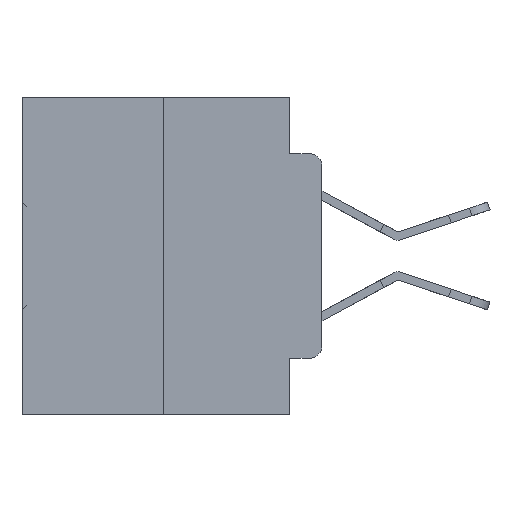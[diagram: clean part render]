
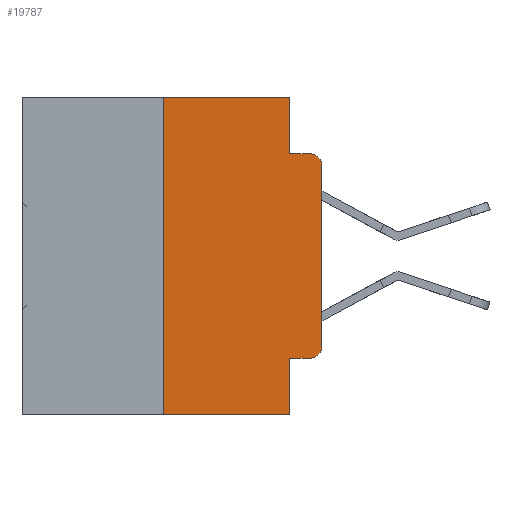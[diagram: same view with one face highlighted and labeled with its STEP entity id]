
A CAD part, left-side view. The second image highlights one B-rep face of the part: STEP entity #19787.
In plain terms, the highlighted planar face has unit normal (-1, 0, 0).
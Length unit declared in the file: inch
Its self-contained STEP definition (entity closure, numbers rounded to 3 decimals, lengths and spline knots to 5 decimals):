
#76 = ORIENTED_EDGE ( 'NONE', *, *, #14428, .T. ) ;
#88 = CARTESIAN_POINT ( 'NONE',  ( 0., 0.051, -0.0885 ) ) ;
#869 = LINE ( 'NONE', #19992, #21057 ) ;
#958 = EDGE_LOOP ( 'NONE', ( #20380, #28626, #30438, #4916, #33759, #33147, #13975, #3211, #12339, #76 ) ) ;
#1133 = VECTOR ( 'NONE', #30900, 39.37008 ) ;
#1187 = CARTESIAN_POINT ( 'NONE',  ( 0., 0.051, 0. ) ) ;
#1416 = DIRECTION ( 'NONE',  ( 0., 0., -1. ) ) ;
#1896 = CARTESIAN_POINT ( 'NONE',  ( 0., 0.02, -0.4115 ) ) ;
#2164 = CARTESIAN_POINT ( 'NONE',  ( 0., 0., -0.3915 ) ) ;
#2449 = CARTESIAN_POINT ( 'NONE',  ( 0., 0.051, 0. ) ) ;
#2727 = DIRECTION ( 'NONE',  ( 0., -1., 0. ) ) ;
#3211 = ORIENTED_EDGE ( 'NONE', *, *, #10693, .F. ) ;
#3385 = CARTESIAN_POINT ( 'NONE',  ( 0., 0.051, -0.4115 ) ) ;
#3514 = VECTOR ( 'NONE', #34036, 39.37008 ) ;
#4916 = ORIENTED_EDGE ( 'NONE', *, *, #24841, .F. ) ;
#5304 = LINE ( 'NONE', #15286, #1133 ) ;
#5607 = CARTESIAN_POINT ( 'NONE',  ( 0., 0.473, -0.5 ) ) ;
#5660 = VERTEX_POINT ( 'NONE', #22393 ) ;
#5994 = AXIS2_PLACEMENT_3D ( 'NONE', #28397, #18089, #31273 ) ;
#7220 = CARTESIAN_POINT ( 'NONE',  ( 0., 0.02, -0.3915 ) ) ;
#7472 = LINE ( 'NONE', #33695, #13221 ) ;
#7655 = DIRECTION ( 'NONE',  ( 0., -1., 0. ) ) ;
#7830 = VERTEX_POINT ( 'NONE', #17586 ) ;
#8299 = EDGE_CURVE ( 'NONE', #16056, #25150, #869, .T. ) ;
#10693 = EDGE_CURVE ( 'NONE', #19736, #5660, #5304, .T. ) ;
#10862 = DIRECTION ( 'NONE',  ( 0., -1., 0. ) ) ;
#11184 = VECTOR ( 'NONE', #10862, 39.37008 ) ;
#11943 = VERTEX_POINT ( 'NONE', #29329 ) ;
#12188 = VERTEX_POINT ( 'NONE', #1896 ) ;
#12197 = EDGE_CURVE ( 'NONE', #22142, #16056, #12635, .T. ) ;
#12215 = EDGE_CURVE ( 'NONE', #23981, #11943, #31503, .T. ) ;
#12339 = ORIENTED_EDGE ( 'NONE', *, *, #21670, .T. ) ;
#12635 = LINE ( 'NONE', #22845, #28660 ) ;
#13221 = VECTOR ( 'NONE', #7655, 39.37008 ) ;
#13975 = ORIENTED_EDGE ( 'NONE', *, *, #24476, .T. ) ;
#14428 = EDGE_CURVE ( 'NONE', #12188, #23981, #33789, .T. ) ;
#14800 = DIRECTION ( 'NONE',  ( -1., 0., 0. ) ) ;
#14894 = CARTESIAN_POINT ( 'NONE',  ( 0., 0.473, 0. ) ) ;
#15049 = EDGE_CURVE ( 'NONE', #20643, #7830, #7472, .T. ) ;
#15286 = CARTESIAN_POINT ( 'NONE',  ( 0., 0.051, 0. ) ) ;
#15921 = CARTESIAN_POINT ( 'NONE',  ( 0., 0.051, -0.4115 ) ) ;
#16056 = VERTEX_POINT ( 'NONE', #31118 ) ;
#16155 = LINE ( 'NONE', #1187, #20629 ) ;
#16492 = AXIS2_PLACEMENT_3D ( 'NONE', #7220, #14800, #1416 ) ;
#17586 = CARTESIAN_POINT ( 'NONE',  ( 0., 0.02, -0.0885 ) ) ;
#17738 = CARTESIAN_POINT ( 'NONE',  ( 0., 0.25, -0.5 ) ) ;
#17887 = FACE_OUTER_BOUND ( 'NONE', #958, .T. ) ;
#18089 = DIRECTION ( 'NONE',  ( -1., 0., 0. ) ) ;
#18784 = EDGE_CURVE ( 'NONE', #11943, #7830, #19951, .T. ) ;
#19736 = VERTEX_POINT ( 'NONE', #3385 ) ;
#19787 = ADVANCED_FACE ( 'NONE', ( #17887 ), #19936, .F. ) ;
#19936 = PLANE ( 'NONE',  #31584 ) ;
#19951 = CIRCLE ( 'NONE', #5994, 0.02 ) ;
#19992 = CARTESIAN_POINT ( 'NONE',  ( 0., 0.473, 0. ) ) ;
#20380 = ORIENTED_EDGE ( 'NONE', *, *, #12215, .T. ) ;
#20629 = VECTOR ( 'NONE', #32931, 39.37008 ) ;
#20643 = VERTEX_POINT ( 'NONE', #88 ) ;
#21057 = VECTOR ( 'NONE', #33093, 39.37008 ) ;
#21670 = EDGE_CURVE ( 'NONE', #19736, #12188, #25962, .T. ) ;
#22142 = VERTEX_POINT ( 'NONE', #17738 ) ;
#22393 = CARTESIAN_POINT ( 'NONE',  ( 0., 0.051, -0.5 ) ) ;
#22575 = DIRECTION ( 'NONE',  ( 0., 0., -1. ) ) ;
#22845 = CARTESIAN_POINT ( 'NONE',  ( 0., 0.25, 0. ) ) ;
#23142 = VECTOR ( 'NONE', #2727, 39.37008 ) ;
#23981 = VERTEX_POINT ( 'NONE', #2164 ) ;
#24040 = DIRECTION ( 'NONE',  ( 0., 0., 1. ) ) ;
#24476 = EDGE_CURVE ( 'NONE', #22142, #5660, #30977, .T. ) ;
#24841 = EDGE_CURVE ( 'NONE', #25150, #20643, #16155, .T. ) ;
#25150 = VERTEX_POINT ( 'NONE', #2449 ) ;
#25210 = DIRECTION ( 'NONE',  ( 1., 0., 0. ) ) ;
#25962 = LINE ( 'NONE', #15921, #11184 ) ;
#28397 = CARTESIAN_POINT ( 'NONE',  ( 0., 0.02, -0.1085 ) ) ;
#28626 = ORIENTED_EDGE ( 'NONE', *, *, #18784, .T. ) ;
#28660 = VECTOR ( 'NONE', #24040, 39.37008 ) ;
#29329 = CARTESIAN_POINT ( 'NONE',  ( 0., 0., -0.1085 ) ) ;
#30438 = ORIENTED_EDGE ( 'NONE', *, *, #15049, .F. ) ;
#30900 = DIRECTION ( 'NONE',  ( 0., 0., -1. ) ) ;
#30977 = LINE ( 'NONE', #5607, #23142 ) ;
#31118 = CARTESIAN_POINT ( 'NONE',  ( 0., 0.25, 0. ) ) ;
#31273 = DIRECTION ( 'NONE',  ( 0., 0., -1. ) ) ;
#31503 = LINE ( 'NONE', #32952, #3514 ) ;
#31584 = AXIS2_PLACEMENT_3D ( 'NONE', #14894, #25210, #22575 ) ;
#32931 = DIRECTION ( 'NONE',  ( 0., 0., -1. ) ) ;
#32952 = CARTESIAN_POINT ( 'NONE',  ( 0., 0., 0. ) ) ;
#33093 = DIRECTION ( 'NONE',  ( 0., -1., 0. ) ) ;
#33147 = ORIENTED_EDGE ( 'NONE', *, *, #12197, .F. ) ;
#33695 = CARTESIAN_POINT ( 'NONE',  ( 0., 0.051, -0.0885 ) ) ;
#33759 = ORIENTED_EDGE ( 'NONE', *, *, #8299, .F. ) ;
#33789 = CIRCLE ( 'NONE', #16492, 0.02 ) ;
#34036 = DIRECTION ( 'NONE',  ( 0., 0., 1. ) ) ;
